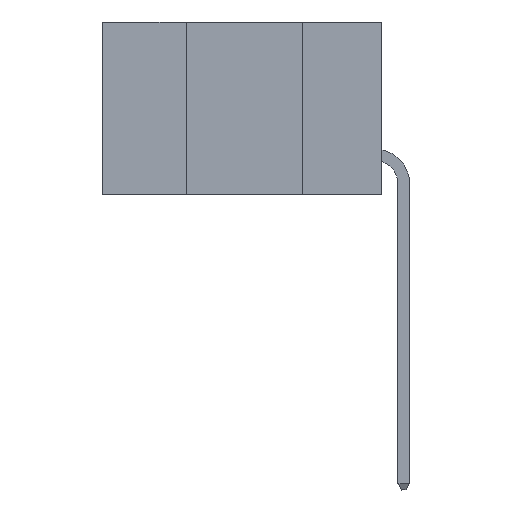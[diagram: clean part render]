
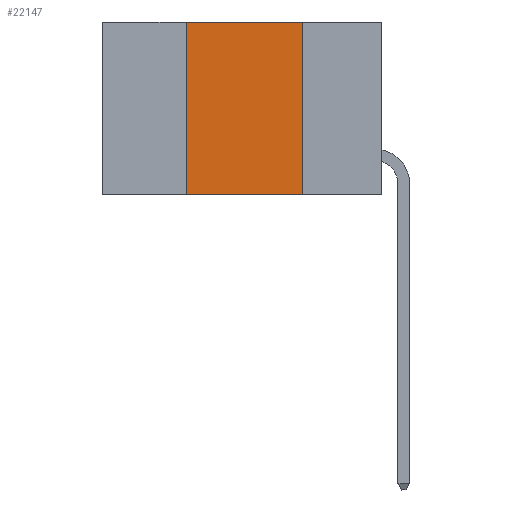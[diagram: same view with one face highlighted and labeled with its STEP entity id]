
A CAD part, left-side view. The second image highlights one B-rep face of the part: STEP entity #22147.
In plain terms, the highlighted planar face has unit normal (-1, 0, 0).
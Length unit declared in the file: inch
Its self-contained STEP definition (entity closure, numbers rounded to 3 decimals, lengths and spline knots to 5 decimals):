
#2501 = EDGE_CURVE ( 'NONE', #30826, #8445, #32433, .T. ) ;
#4857 = VERTEX_POINT ( 'NONE', #49599 ) ;
#5500 = CARTESIAN_POINT ( 'NONE',  ( 0., 0.42, 0. ) ) ;
#8445 = VERTEX_POINT ( 'NONE', #45389 ) ;
#10508 = ORIENTED_EDGE ( 'NONE', *, *, #2501, .F. ) ;
#12232 = ORIENTED_EDGE ( 'NONE', *, *, #40819, .T. ) ;
#13230 = LINE ( 'NONE', #18244, #16335 ) ;
#13437 = DIRECTION ( 'NONE',  ( 0., 0., -1. ) ) ;
#13532 = DIRECTION ( 'NONE',  ( 0., 0., 1. ) ) ;
#16335 = VECTOR ( 'NONE', #42065, 39.37008 ) ;
#18244 = CARTESIAN_POINT ( 'NONE',  ( 0., 0.6, -0.37 ) ) ;
#18401 = CARTESIAN_POINT ( 'NONE',  ( 0., 0.6, 0. ) ) ;
#19113 = VECTOR ( 'NONE', #13437, 39.37008 ) ;
#19691 = VECTOR ( 'NONE', #13532, 39.37008 ) ;
#21584 = LINE ( 'NONE', #44964, #19113 ) ;
#21870 = DIRECTION ( 'NONE',  ( 1., 0., 0. ) ) ;
#22147 = ADVANCED_FACE ( 'NONE', ( #45575 ), #41547, .F. ) ;
#23053 = CARTESIAN_POINT ( 'NONE',  ( 0., 0.42, 0. ) ) ;
#23465 = VERTEX_POINT ( 'NONE', #42221 ) ;
#25410 = ORIENTED_EDGE ( 'NONE', *, *, #37502, .F. ) ;
#27082 = AXIS2_PLACEMENT_3D ( 'NONE', #18401, #21870, #38232 ) ;
#30148 = LINE ( 'NONE', #5500, #19691 ) ;
#30826 = VERTEX_POINT ( 'NONE', #23053 ) ;
#32433 = LINE ( 'NONE', #35332, #36166 ) ;
#35332 = CARTESIAN_POINT ( 'NONE',  ( 0., 0.6, 0. ) ) ;
#36166 = VECTOR ( 'NONE', #39481, 39.37008 ) ;
#36376 = EDGE_LOOP ( 'NONE', ( #25410, #10508, #47351, #12232 ) ) ;
#37502 = EDGE_CURVE ( 'NONE', #8445, #23465, #21584, .T. ) ;
#38232 = DIRECTION ( 'NONE',  ( 0., 0., -1. ) ) ;
#39481 = DIRECTION ( 'NONE',  ( 0., -1., 0. ) ) ;
#40819 = EDGE_CURVE ( 'NONE', #4857, #23465, #13230, .T. ) ;
#41547 = PLANE ( 'NONE',  #27082 ) ;
#42065 = DIRECTION ( 'NONE',  ( 0., -1., 0. ) ) ;
#42221 = CARTESIAN_POINT ( 'NONE',  ( 0., 0.17, -0.37 ) ) ;
#44964 = CARTESIAN_POINT ( 'NONE',  ( 0., 0.17, 0. ) ) ;
#45389 = CARTESIAN_POINT ( 'NONE',  ( 0., 0.17, 0. ) ) ;
#45575 = FACE_OUTER_BOUND ( 'NONE', #36376, .T. ) ;
#47351 = ORIENTED_EDGE ( 'NONE', *, *, #47497, .F. ) ;
#47497 = EDGE_CURVE ( 'NONE', #4857, #30826, #30148, .T. ) ;
#49599 = CARTESIAN_POINT ( 'NONE',  ( 0., 0.42, -0.37 ) ) ;
